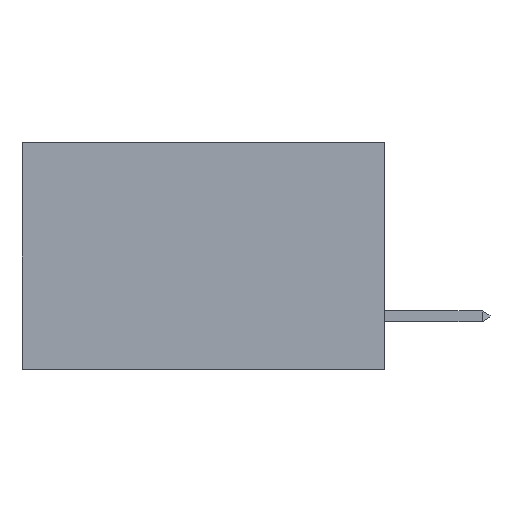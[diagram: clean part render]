
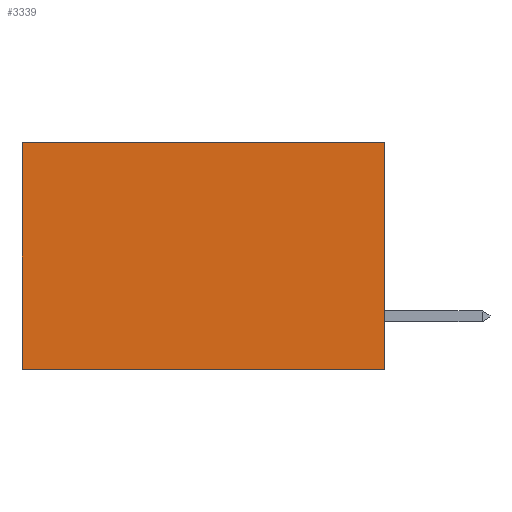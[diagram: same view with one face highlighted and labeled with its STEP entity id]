
A CAD part, left-side view. The second image highlights one B-rep face of the part: STEP entity #3339.
In plain terms, the highlighted planar face has unit normal (-1, 0, 0).
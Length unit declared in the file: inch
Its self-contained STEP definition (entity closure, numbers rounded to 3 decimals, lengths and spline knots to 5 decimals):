
#156 = CARTESIAN_POINT ( 'NONE',  ( 0.2875, 0., -0.375 ) ) ;
#224 = VERTEX_POINT ( 'NONE', #8613 ) ;
#283 = DIRECTION ( 'NONE',  ( 0., 0., -1. ) ) ;
#457 = CARTESIAN_POINT ( 'NONE',  ( 0.2875, 0.6, -0.375 ) ) ;
#589 = CARTESIAN_POINT ( 'NONE',  ( 0.2875, 0., 0. ) ) ;
#777 = VERTEX_POINT ( 'NONE', #5313 ) ;
#950 = ORIENTED_EDGE ( 'NONE', *, *, #12811, .F. ) ;
#1067 = EDGE_CURVE ( 'NONE', #1792, #3946, #2085, .T. ) ;
#1102 = DIRECTION ( 'NONE',  ( 0., 0., -1. ) ) ;
#1445 = DIRECTION ( 'NONE',  ( 0., 0., -1. ) ) ;
#1792 = VERTEX_POINT ( 'NONE', #8568 ) ;
#1920 = VECTOR ( 'NONE', #1102, 39.37008 ) ;
#2065 = EDGE_LOOP ( 'NONE', ( #7062, #950, #6697, #8723 ) ) ;
#2085 = LINE ( 'NONE', #6100, #1920 ) ;
#3303 = DIRECTION ( 'NONE',  ( 1., 0., 0. ) ) ;
#3339 = ADVANCED_FACE ( 'NONE', ( #9161 ), #12327, .F. ) ;
#3946 = VERTEX_POINT ( 'NONE', #12434 ) ;
#4116 = CARTESIAN_POINT ( 'NONE',  ( 0.2875, 0., -0.375 ) ) ;
#5313 = CARTESIAN_POINT ( 'NONE',  ( 0.2875, 0.6, -0.375 ) ) ;
#5316 = VECTOR ( 'NONE', #1445, 39.37008 ) ;
#5910 = EDGE_CURVE ( 'NONE', #224, #777, #6435, .T. ) ;
#6100 = CARTESIAN_POINT ( 'NONE',  ( 0.2875, 0., -0.375 ) ) ;
#6278 = LINE ( 'NONE', #4116, #9375 ) ;
#6435 = LINE ( 'NONE', #457, #5316 ) ;
#6697 = ORIENTED_EDGE ( 'NONE', *, *, #1067, .F. ) ;
#7062 = ORIENTED_EDGE ( 'NONE', *, *, #5910, .T. ) ;
#7111 = EDGE_CURVE ( 'NONE', #1792, #224, #11580, .T. ) ;
#8568 = CARTESIAN_POINT ( 'NONE',  ( 0.2875, 0., 0. ) ) ;
#8613 = CARTESIAN_POINT ( 'NONE',  ( 0.2875, 0.6, 0. ) ) ;
#8723 = ORIENTED_EDGE ( 'NONE', *, *, #7111, .T. ) ;
#9077 = AXIS2_PLACEMENT_3D ( 'NONE', #156, #3303, #283 ) ;
#9161 = FACE_OUTER_BOUND ( 'NONE', #2065, .T. ) ;
#9375 = VECTOR ( 'NONE', #10302, 39.37008 ) ;
#10302 = DIRECTION ( 'NONE',  ( 0., 1., 0. ) ) ;
#10337 = DIRECTION ( 'NONE',  ( 0., 1., 0. ) ) ;
#11194 = VECTOR ( 'NONE', #10337, 39.37008 ) ;
#11580 = LINE ( 'NONE', #589, #11194 ) ;
#12327 = PLANE ( 'NONE',  #9077 ) ;
#12434 = CARTESIAN_POINT ( 'NONE',  ( 0.2875, 0., -0.375 ) ) ;
#12811 = EDGE_CURVE ( 'NONE', #3946, #777, #6278, .T. ) ;
